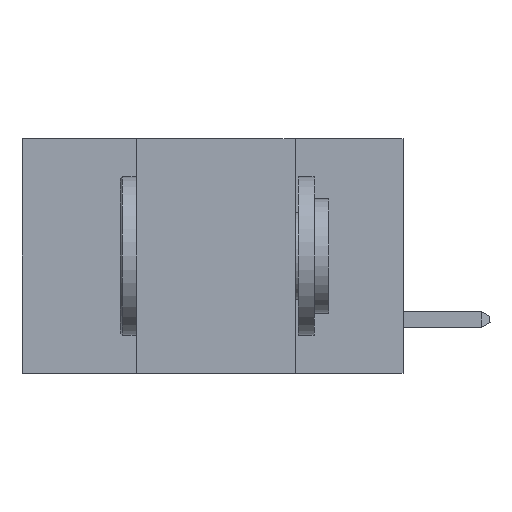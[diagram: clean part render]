
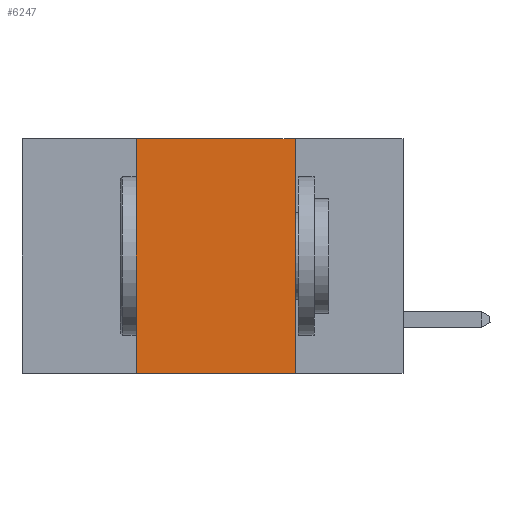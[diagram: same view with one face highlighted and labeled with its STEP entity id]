
A CAD part, left-side view. The second image highlights one B-rep face of the part: STEP entity #6247.
In plain terms, the highlighted planar face has unit normal (-1, 0, 0).
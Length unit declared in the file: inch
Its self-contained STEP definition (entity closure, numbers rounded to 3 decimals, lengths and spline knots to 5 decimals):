
#16 = CARTESIAN_POINT ( 'NONE',  ( 0., 0.17, -0.37 ) ) ;
#196 = LINE ( 'NONE', #5936, #9212 ) ;
#674 = LINE ( 'NONE', #4164, #9687 ) ;
#1545 = LINE ( 'NONE', #2123, #16058 ) ;
#2123 = CARTESIAN_POINT ( 'NONE',  ( 0., 0.42, 0. ) ) ;
#2196 = CARTESIAN_POINT ( 'NONE',  ( 0., 0.6, 0. ) ) ;
#3383 = CARTESIAN_POINT ( 'NONE',  ( 0., 0.42, -0.37 ) ) ;
#3467 = CARTESIAN_POINT ( 'NONE',  ( 0., 0.17, 0. ) ) ;
#4100 = DIRECTION ( 'NONE',  ( 0., 0., -1. ) ) ;
#4164 = CARTESIAN_POINT ( 'NONE',  ( 0., 0.17, 0. ) ) ;
#5118 = DIRECTION ( 'NONE',  ( 0., 0., -1. ) ) ;
#5564 = FACE_OUTER_BOUND ( 'NONE', #10578, .T. ) ;
#5672 = VERTEX_POINT ( 'NONE', #3467 ) ;
#5730 = EDGE_CURVE ( 'NONE', #17899, #17688, #13460, .T. ) ;
#5936 = CARTESIAN_POINT ( 'NONE',  ( 0., 0.6, 0. ) ) ;
#6247 = ADVANCED_FACE ( 'NONE', ( #5564 ), #17639, .F. ) ;
#6780 = EDGE_CURVE ( 'NONE', #17899, #14294, #1545, .T. ) ;
#7674 = DIRECTION ( 'NONE',  ( 0., 0., 1. ) ) ;
#8019 = CARTESIAN_POINT ( 'NONE',  ( 0., 0.6, -0.37 ) ) ;
#8941 = AXIS2_PLACEMENT_3D ( 'NONE', #2196, #12039, #5118 ) ;
#9212 = VECTOR ( 'NONE', #17229, 39.37008 ) ;
#9687 = VECTOR ( 'NONE', #4100, 39.37008 ) ;
#10152 = ORIENTED_EDGE ( 'NONE', *, *, #16586, .F. ) ;
#10577 = EDGE_CURVE ( 'NONE', #14294, #5672, #196, .T. ) ;
#10578 = EDGE_LOOP ( 'NONE', ( #10152, #14068, #15744, #13192 ) ) ;
#10747 = CARTESIAN_POINT ( 'NONE',  ( 0., 0.42, 0. ) ) ;
#11065 = VECTOR ( 'NONE', #13822, 39.37008 ) ;
#12039 = DIRECTION ( 'NONE',  ( 1., 0., 0. ) ) ;
#13192 = ORIENTED_EDGE ( 'NONE', *, *, #5730, .T. ) ;
#13460 = LINE ( 'NONE', #8019, #11065 ) ;
#13822 = DIRECTION ( 'NONE',  ( 0., -1., 0. ) ) ;
#14068 = ORIENTED_EDGE ( 'NONE', *, *, #10577, .F. ) ;
#14294 = VERTEX_POINT ( 'NONE', #10747 ) ;
#15744 = ORIENTED_EDGE ( 'NONE', *, *, #6780, .F. ) ;
#16058 = VECTOR ( 'NONE', #7674, 39.37008 ) ;
#16586 = EDGE_CURVE ( 'NONE', #5672, #17688, #674, .T. ) ;
#17229 = DIRECTION ( 'NONE',  ( 0., -1., 0. ) ) ;
#17639 = PLANE ( 'NONE',  #8941 ) ;
#17688 = VERTEX_POINT ( 'NONE', #16 ) ;
#17899 = VERTEX_POINT ( 'NONE', #3383 ) ;
